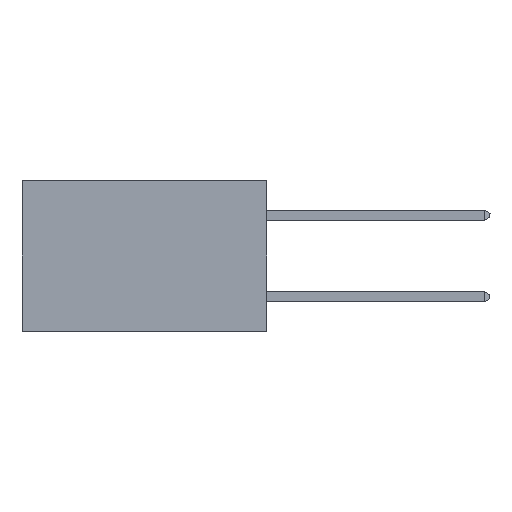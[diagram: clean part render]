
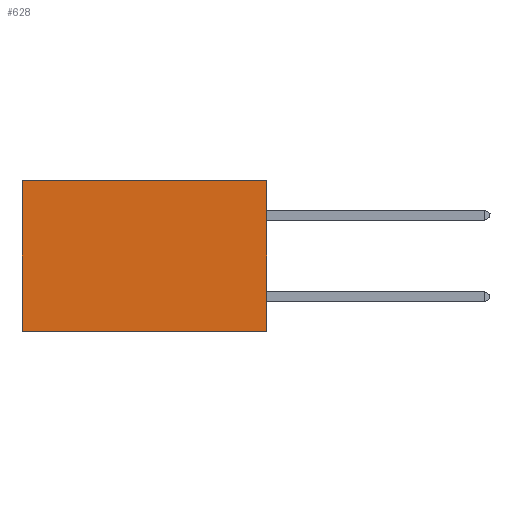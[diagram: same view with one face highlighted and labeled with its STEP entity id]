
A CAD part, left-side view. The second image highlights one B-rep face of the part: STEP entity #628.
In plain terms, the highlighted planar face has unit normal (-1, 0, 0).
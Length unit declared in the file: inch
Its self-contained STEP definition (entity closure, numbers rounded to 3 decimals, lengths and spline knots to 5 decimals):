
#346 = DIRECTION ( 'NONE',  ( 0., 1., 0. ) ) ;
#449 = VECTOR ( 'NONE', #4770, 39.37008 ) ;
#504 = CARTESIAN_POINT ( 'NONE',  ( 0.2875, 0., -0.37 ) ) ;
#539 = EDGE_LOOP ( 'NONE', ( #5016, #2770, #19225, #4339 ) ) ;
#628 = ADVANCED_FACE ( 'NONE', ( #1752 ), #19321, .F. ) ;
#1752 = FACE_OUTER_BOUND ( 'NONE', #539, .T. ) ;
#2212 = LINE ( 'NONE', #504, #14770 ) ;
#2219 = CARTESIAN_POINT ( 'NONE',  ( 0.2875, 0., 0. ) ) ;
#2770 = ORIENTED_EDGE ( 'NONE', *, *, #3833, .F. ) ;
#3280 = CARTESIAN_POINT ( 'NONE',  ( 0.2875, 0., 0. ) ) ;
#3319 = CARTESIAN_POINT ( 'NONE',  ( 0.2875, 0.6, -0.37 ) ) ;
#3541 = VECTOR ( 'NONE', #9492, 39.37008 ) ;
#3833 = EDGE_CURVE ( 'NONE', #16518, #20061, #2212, .T. ) ;
#4339 = ORIENTED_EDGE ( 'NONE', *, *, #6290, .T. ) ;
#4770 = DIRECTION ( 'NONE',  ( 0., 1., 0. ) ) ;
#5016 = ORIENTED_EDGE ( 'NONE', *, *, #5511, .T. ) ;
#5119 = EDGE_CURVE ( 'NONE', #8547, #16518, #21658, .T. ) ;
#5511 = EDGE_CURVE ( 'NONE', #6849, #20061, #17125, .T. ) ;
#6290 = EDGE_CURVE ( 'NONE', #8547, #6849, #10206, .T. ) ;
#6849 = VERTEX_POINT ( 'NONE', #16455 ) ;
#7082 = VECTOR ( 'NONE', #16908, 39.37008 ) ;
#8547 = VERTEX_POINT ( 'NONE', #2219 ) ;
#9492 = DIRECTION ( 'NONE',  ( 0., 0., -1. ) ) ;
#9819 = CARTESIAN_POINT ( 'NONE',  ( 0.2875, 0., -0.37 ) ) ;
#10206 = LINE ( 'NONE', #13221, #449 ) ;
#13221 = CARTESIAN_POINT ( 'NONE',  ( 0.2875, 0., 0. ) ) ;
#13340 = AXIS2_PLACEMENT_3D ( 'NONE', #19482, #19250, #19244 ) ;
#14770 = VECTOR ( 'NONE', #346, 39.37008 ) ;
#16455 = CARTESIAN_POINT ( 'NONE',  ( 0.2875, 0.6, 0. ) ) ;
#16518 = VERTEX_POINT ( 'NONE', #9819 ) ;
#16908 = DIRECTION ( 'NONE',  ( 0., 0., -1. ) ) ;
#17125 = LINE ( 'NONE', #17961, #3541 ) ;
#17961 = CARTESIAN_POINT ( 'NONE',  ( 0.2875, 0.6, 0. ) ) ;
#19225 = ORIENTED_EDGE ( 'NONE', *, *, #5119, .F. ) ;
#19244 = DIRECTION ( 'NONE',  ( 0., 0., -1. ) ) ;
#19250 = DIRECTION ( 'NONE',  ( 1., 0., 0. ) ) ;
#19321 = PLANE ( 'NONE',  #13340 ) ;
#19482 = CARTESIAN_POINT ( 'NONE',  ( 0.2875, 0., 0. ) ) ;
#20061 = VERTEX_POINT ( 'NONE', #3319 ) ;
#21658 = LINE ( 'NONE', #3280, #7082 ) ;
